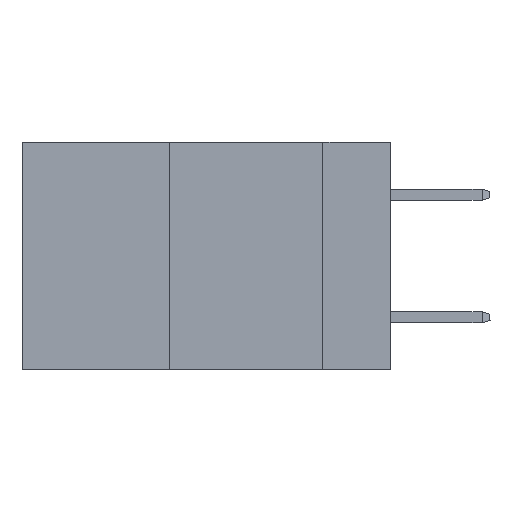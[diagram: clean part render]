
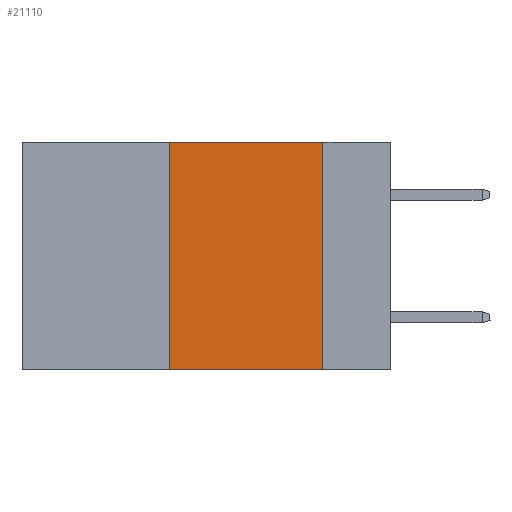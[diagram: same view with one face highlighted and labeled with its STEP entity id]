
A CAD part, left-side view. The second image highlights one B-rep face of the part: STEP entity #21110.
In plain terms, the highlighted planar face has unit normal (-1, 0, 0).
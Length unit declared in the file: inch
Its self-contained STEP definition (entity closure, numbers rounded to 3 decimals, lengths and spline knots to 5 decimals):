
#361 = DIRECTION ( 'NONE',  ( 0., 0., -1. ) ) ;
#536 = ORIENTED_EDGE ( 'NONE', *, *, #11014, .T. ) ;
#3135 = CARTESIAN_POINT ( 'NONE',  ( 0., 0.11, -0.37 ) ) ;
#3198 = VERTEX_POINT ( 'NONE', #3135 ) ;
#3665 = DIRECTION ( 'NONE',  ( 0., -1., 0. ) ) ;
#3926 = VECTOR ( 'NONE', #4839, 39.37008 ) ;
#4098 = LINE ( 'NONE', #13336, #12596 ) ;
#4839 = DIRECTION ( 'NONE',  ( 0., -1., 0. ) ) ;
#5023 = LINE ( 'NONE', #8161, #3926 ) ;
#5637 = EDGE_CURVE ( 'NONE', #12485, #19528, #5023, .T. ) ;
#5861 = EDGE_LOOP ( 'NONE', ( #17617, #14163, #9238, #536 ) ) ;
#6837 = EDGE_CURVE ( 'NONE', #19528, #3198, #20460, .T. ) ;
#7032 = CARTESIAN_POINT ( 'NONE',  ( 0., 0.6, -0.37 ) ) ;
#7405 = CARTESIAN_POINT ( 'NONE',  ( 0., 0.36, 0. ) ) ;
#7652 = FACE_OUTER_BOUND ( 'NONE', #5861, .T. ) ;
#8161 = CARTESIAN_POINT ( 'NONE',  ( 0., 0.6, 0. ) ) ;
#8783 = VECTOR ( 'NONE', #3665, 39.37008 ) ;
#9028 = PLANE ( 'NONE',  #21136 ) ;
#9238 = ORIENTED_EDGE ( 'NONE', *, *, #14710, .F. ) ;
#9613 = CARTESIAN_POINT ( 'NONE',  ( 0., 0.36, -0.37 ) ) ;
#10289 = CARTESIAN_POINT ( 'NONE',  ( 0., 0.11, 0. ) ) ;
#10725 = DIRECTION ( 'NONE',  ( 1., 0., 0. ) ) ;
#11014 = EDGE_CURVE ( 'NONE', #13906, #3198, #13261, .T. ) ;
#11065 = VECTOR ( 'NONE', #11977, 39.37008 ) ;
#11977 = DIRECTION ( 'NONE',  ( 0., 0., -1. ) ) ;
#12354 = CARTESIAN_POINT ( 'NONE',  ( 0., 0.11, 0. ) ) ;
#12485 = VERTEX_POINT ( 'NONE', #7405 ) ;
#12596 = VECTOR ( 'NONE', #15036, 39.37008 ) ;
#13261 = LINE ( 'NONE', #7032, #8783 ) ;
#13336 = CARTESIAN_POINT ( 'NONE',  ( 0., 0.36, 0. ) ) ;
#13906 = VERTEX_POINT ( 'NONE', #9613 ) ;
#14030 = CARTESIAN_POINT ( 'NONE',  ( 0., 0.6, 0. ) ) ;
#14163 = ORIENTED_EDGE ( 'NONE', *, *, #5637, .F. ) ;
#14710 = EDGE_CURVE ( 'NONE', #13906, #12485, #4098, .T. ) ;
#15036 = DIRECTION ( 'NONE',  ( 0., 0., 1. ) ) ;
#17617 = ORIENTED_EDGE ( 'NONE', *, *, #6837, .F. ) ;
#19528 = VERTEX_POINT ( 'NONE', #12354 ) ;
#20460 = LINE ( 'NONE', #10289, #11065 ) ;
#21110 = ADVANCED_FACE ( 'NONE', ( #7652 ), #9028, .F. ) ;
#21136 = AXIS2_PLACEMENT_3D ( 'NONE', #14030, #10725, #361 ) ;
